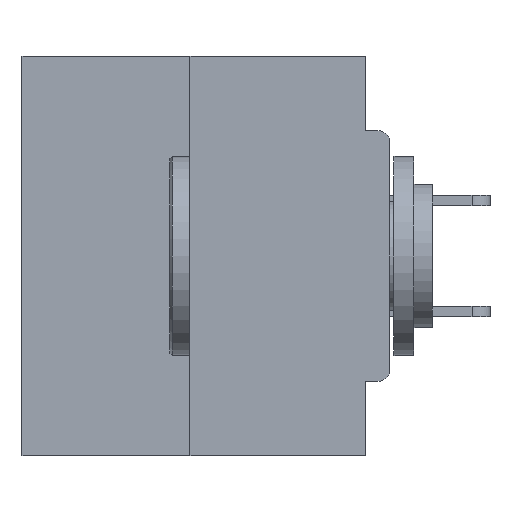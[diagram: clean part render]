
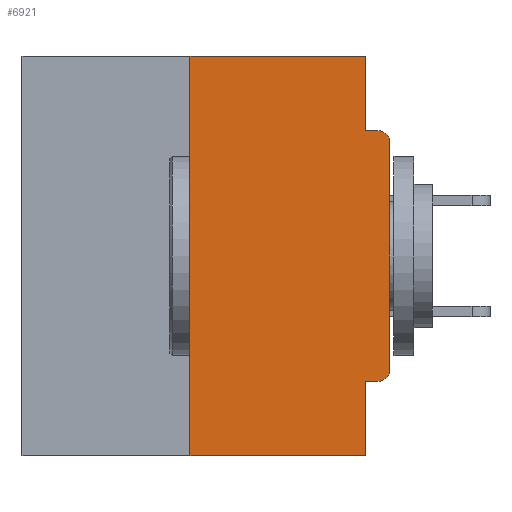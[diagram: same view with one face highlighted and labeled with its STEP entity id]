
A CAD part, left-side view. The second image highlights one B-rep face of the part: STEP entity #6921.
In plain terms, the highlighted planar face has unit normal (-1, 0, 0).
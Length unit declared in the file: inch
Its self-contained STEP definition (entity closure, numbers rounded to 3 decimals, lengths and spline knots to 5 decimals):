
#165 = EDGE_CURVE ( 'NONE', #31499, #35355, #19375, .T. ) ;
#223 = CARTESIAN_POINT ( 'NONE',  ( 0., 0., -0.1085 ) ) ;
#748 = VERTEX_POINT ( 'NONE', #42630 ) ;
#1533 = CIRCLE ( 'NONE', #33530, 0.015 ) ;
#1583 = VECTOR ( 'NONE', #1719, 39.37008 ) ;
#1588 = EDGE_CURVE ( 'NONE', #3232, #9503, #1533, .T. ) ;
#1591 = DIRECTION ( 'NONE',  ( -1., 0., 0. ) ) ;
#1719 = DIRECTION ( 'NONE',  ( 0., -1., 0. ) ) ;
#2658 = DIRECTION ( 'NONE',  ( -1., 0., 0. ) ) ;
#3232 = VERTEX_POINT ( 'NONE', #223 ) ;
#3625 = CARTESIAN_POINT ( 'NONE',  ( 0., 0.031, 0. ) ) ;
#5167 = DIRECTION ( 'NONE',  ( 0., 0., -1. ) ) ;
#5670 = EDGE_CURVE ( 'NONE', #35355, #14604, #35954, .T. ) ;
#6304 = EDGE_CURVE ( 'NONE', #14604, #9503, #17145, .T. ) ;
#6337 = VERTEX_POINT ( 'NONE', #18962 ) ;
#6646 = DIRECTION ( 'NONE',  ( 0., 0., -1. ) ) ;
#6892 = LINE ( 'NONE', #28508, #33177 ) ;
#6921 = ADVANCED_FACE ( 'NONE', ( #21369 ), #28751, .F. ) ;
#7356 = ORIENTED_EDGE ( 'NONE', *, *, #22617, .F. ) ;
#9135 = CARTESIAN_POINT ( 'NONE',  ( 0., 0.015, -0.1085 ) ) ;
#9503 = VERTEX_POINT ( 'NONE', #25741 ) ;
#10202 = VECTOR ( 'NONE', #30004, 39.37008 ) ;
#11627 = CARTESIAN_POINT ( 'NONE',  ( 0., 0.46, 0. ) ) ;
#12406 = AXIS2_PLACEMENT_3D ( 'NONE', #22113, #1591, #5167 ) ;
#13099 = DIRECTION ( 'NONE',  ( 0., 1., 0. ) ) ;
#13713 = CARTESIAN_POINT ( 'NONE',  ( 0., 0.46, 0. ) ) ;
#14588 = EDGE_CURVE ( 'NONE', #23424, #17511, #32620, .T. ) ;
#14604 = VERTEX_POINT ( 'NONE', #20601 ) ;
#15111 = DIRECTION ( 'NONE',  ( 0., 0., 1. ) ) ;
#15483 = ORIENTED_EDGE ( 'NONE', *, *, #40805, .F. ) ;
#16042 = ORIENTED_EDGE ( 'NONE', *, *, #39057, .T. ) ;
#16188 = CARTESIAN_POINT ( 'NONE',  ( 0., 0., 0. ) ) ;
#16367 = ORIENTED_EDGE ( 'NONE', *, *, #27832, .T. ) ;
#16468 = DIRECTION ( 'NONE',  ( 0., 0., -1. ) ) ;
#16673 = LINE ( 'NONE', #16188, #10202 ) ;
#17145 = LINE ( 'NONE', #28870, #1583 ) ;
#17329 = DIRECTION ( 'NONE',  ( 0., -1., 0. ) ) ;
#17511 = VERTEX_POINT ( 'NONE', #37475 ) ;
#17679 = EDGE_LOOP ( 'NONE', ( #25376, #7356, #16367, #15483, #37694, #16042, #26330, #37276, #40647, #42827 ) ) ;
#18962 = CARTESIAN_POINT ( 'NONE',  ( 0., 0.25, -0.5 ) ) ;
#19375 = LINE ( 'NONE', #13713, #30111 ) ;
#20601 = CARTESIAN_POINT ( 'NONE',  ( 0., 0.031, -0.0935 ) ) ;
#21045 = AXIS2_PLACEMENT_3D ( 'NONE', #11627, #32345, #38490 ) ;
#21369 = FACE_OUTER_BOUND ( 'NONE', #17679, .T. ) ;
#22030 = VERTEX_POINT ( 'NONE', #29803 ) ;
#22113 = CARTESIAN_POINT ( 'NONE',  ( 0., 0.015, -0.3915 ) ) ;
#22535 = CIRCLE ( 'NONE', #12406, 0.015 ) ;
#22617 = EDGE_CURVE ( 'NONE', #6337, #31499, #25362, .T. ) ;
#23424 = VERTEX_POINT ( 'NONE', #43839 ) ;
#24073 = CARTESIAN_POINT ( 'NONE',  ( 0., 0.46, -0.5 ) ) ;
#24152 = EDGE_CURVE ( 'NONE', #22030, #3232, #16673, .T. ) ;
#25200 = DIRECTION ( 'NONE',  ( 0., 0., -1. ) ) ;
#25362 = LINE ( 'NONE', #35662, #41453 ) ;
#25376 = ORIENTED_EDGE ( 'NONE', *, *, #165, .F. ) ;
#25741 = CARTESIAN_POINT ( 'NONE',  ( 0., 0.015, -0.0935 ) ) ;
#25773 = VECTOR ( 'NONE', #6646, 39.37008 ) ;
#26330 = ORIENTED_EDGE ( 'NONE', *, *, #24152, .T. ) ;
#26767 = CARTESIAN_POINT ( 'NONE',  ( 0., 0., -0.4065 ) ) ;
#27130 = VECTOR ( 'NONE', #17329, 39.37008 ) ;
#27832 = EDGE_CURVE ( 'NONE', #6337, #748, #43791, .T. ) ;
#28508 = CARTESIAN_POINT ( 'NONE',  ( 0., 0.031, -0.5 ) ) ;
#28751 = PLANE ( 'NONE',  #21045 ) ;
#28870 = CARTESIAN_POINT ( 'NONE',  ( 0., 0., -0.0935 ) ) ;
#29803 = CARTESIAN_POINT ( 'NONE',  ( 0., 0., -0.3915 ) ) ;
#30004 = DIRECTION ( 'NONE',  ( 0., 0., 1. ) ) ;
#30105 = CARTESIAN_POINT ( 'NONE',  ( 0., 0.031, 0. ) ) ;
#30111 = VECTOR ( 'NONE', #42690, 39.37008 ) ;
#31499 = VERTEX_POINT ( 'NONE', #32729 ) ;
#32345 = DIRECTION ( 'NONE',  ( 1., 0., 0. ) ) ;
#32620 = LINE ( 'NONE', #26767, #33114 ) ;
#32729 = CARTESIAN_POINT ( 'NONE',  ( 0., 0.25, 0. ) ) ;
#33114 = VECTOR ( 'NONE', #13099, 39.37008 ) ;
#33177 = VECTOR ( 'NONE', #25200, 39.37008 ) ;
#33530 = AXIS2_PLACEMENT_3D ( 'NONE', #9135, #2658, #16468 ) ;
#35355 = VERTEX_POINT ( 'NONE', #30105 ) ;
#35662 = CARTESIAN_POINT ( 'NONE',  ( 0., 0.25, 0. ) ) ;
#35954 = LINE ( 'NONE', #3625, #25773 ) ;
#37276 = ORIENTED_EDGE ( 'NONE', *, *, #1588, .T. ) ;
#37475 = CARTESIAN_POINT ( 'NONE',  ( 0., 0.031, -0.4065 ) ) ;
#37694 = ORIENTED_EDGE ( 'NONE', *, *, #14588, .F. ) ;
#38490 = DIRECTION ( 'NONE',  ( 0., 0., -1. ) ) ;
#39057 = EDGE_CURVE ( 'NONE', #23424, #22030, #22535, .T. ) ;
#40647 = ORIENTED_EDGE ( 'NONE', *, *, #6304, .F. ) ;
#40805 = EDGE_CURVE ( 'NONE', #17511, #748, #6892, .T. ) ;
#41453 = VECTOR ( 'NONE', #15111, 39.37008 ) ;
#42630 = CARTESIAN_POINT ( 'NONE',  ( 0., 0.031, -0.5 ) ) ;
#42690 = DIRECTION ( 'NONE',  ( 0., -1., 0. ) ) ;
#42827 = ORIENTED_EDGE ( 'NONE', *, *, #5670, .F. ) ;
#43791 = LINE ( 'NONE', #24073, #27130 ) ;
#43839 = CARTESIAN_POINT ( 'NONE',  ( 0., 0.015, -0.4065 ) ) ;
